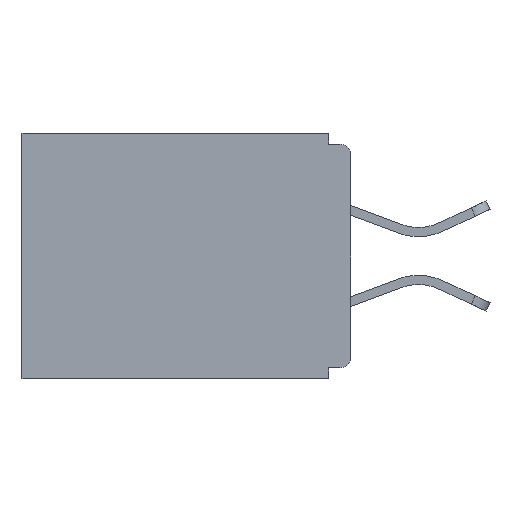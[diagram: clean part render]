
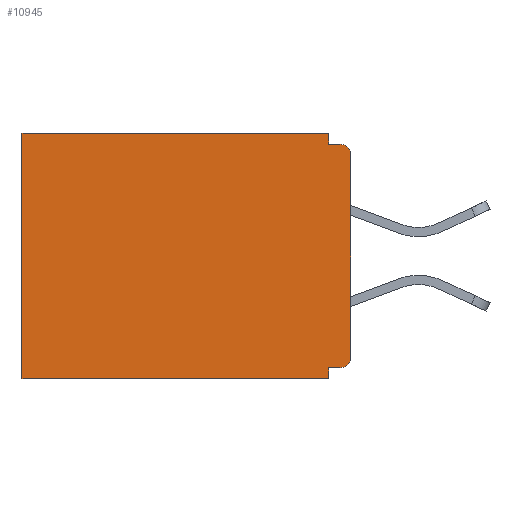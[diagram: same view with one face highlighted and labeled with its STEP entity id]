
A CAD part, left-side view. The second image highlights one B-rep face of the part: STEP entity #10945.
In plain terms, the highlighted planar face has unit normal (-1, 0, 0).
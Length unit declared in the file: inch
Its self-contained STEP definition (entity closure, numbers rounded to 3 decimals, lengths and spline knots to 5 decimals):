
#43 = AXIS2_PLACEMENT_3D ( 'NONE', #18187, #20463, #11558 ) ;
#1147 = CARTESIAN_POINT ( 'NONE',  ( 0.298, 0., -0.343 ) ) ;
#1182 = LINE ( 'NONE', #28851, #17991 ) ;
#1519 = EDGE_CURVE ( 'NONE', #20326, #28762, #3166, .T. ) ;
#1587 = LINE ( 'NONE', #18025, #18782 ) ;
#1724 = ORIENTED_EDGE ( 'NONE', *, *, #22339, .F. ) ;
#2515 = DIRECTION ( 'NONE',  ( 0., 0., -1. ) ) ;
#3166 = LINE ( 'NONE', #6079, #15088 ) ;
#3562 = LINE ( 'NONE', #15911, #8822 ) ;
#3618 = VECTOR ( 'NONE', #20977, 39.37008 ) ;
#3961 = ORIENTED_EDGE ( 'NONE', *, *, #25768, .F. ) ;
#4178 = CARTESIAN_POINT ( 'NONE',  ( 0.298, 0.46, 0. ) ) ;
#4232 = EDGE_CURVE ( 'NONE', #9191, #28944, #1587, .T. ) ;
#4562 = CARTESIAN_POINT ( 'NONE',  ( 0.298, 0.015, -0.328 ) ) ;
#4910 = CARTESIAN_POINT ( 'NONE',  ( 0.298, 0.46, -0.343 ) ) ;
#5823 = ORIENTED_EDGE ( 'NONE', *, *, #20097, .F. ) ;
#6053 = LINE ( 'NONE', #25702, #3618 ) ;
#6079 = CARTESIAN_POINT ( 'NONE',  ( 0.298, 0., 0. ) ) ;
#6229 = DIRECTION ( 'NONE',  ( -1., 0., 0. ) ) ;
#6431 = VERTEX_POINT ( 'NONE', #21099 ) ;
#6627 = DIRECTION ( 'NONE',  ( 0., 0., -1. ) ) ;
#6836 = EDGE_CURVE ( 'NONE', #28762, #16890, #15283, .T. ) ;
#7555 = EDGE_LOOP ( 'NONE', ( #28119, #8310, #25436, #8797, #10883, #5823, #1724, #18919, #17850, #3961 ) ) ;
#7641 = VECTOR ( 'NONE', #24606, 39.37008 ) ;
#7887 = VECTOR ( 'NONE', #7920, 39.37008 ) ;
#7920 = DIRECTION ( 'NONE',  ( 0., 1., 0. ) ) ;
#7973 = EDGE_CURVE ( 'NONE', #12589, #15435, #6053, .T. ) ;
#8310 = ORIENTED_EDGE ( 'NONE', *, *, #7973, .F. ) ;
#8620 = DIRECTION ( 'NONE',  ( 0., 0., -1. ) ) ;
#8695 = CARTESIAN_POINT ( 'NONE',  ( 0.298, 0.031, 0. ) ) ;
#8797 = ORIENTED_EDGE ( 'NONE', *, *, #1519, .T. ) ;
#8822 = VECTOR ( 'NONE', #2515, 39.37008 ) ;
#9191 = VERTEX_POINT ( 'NONE', #4562 ) ;
#10883 = ORIENTED_EDGE ( 'NONE', *, *, #6836, .T. ) ;
#10903 = CARTESIAN_POINT ( 'NONE',  ( 0.298, 0.015, -0.015 ) ) ;
#10945 = ADVANCED_FACE ( 'NONE', ( #22767 ), #12918, .F. ) ;
#10976 = CARTESIAN_POINT ( 'NONE',  ( 0.298, 0.015, -0.313 ) ) ;
#11558 = DIRECTION ( 'NONE',  ( 0., 0., -1. ) ) ;
#12589 = VERTEX_POINT ( 'NONE', #26981 ) ;
#12918 = PLANE ( 'NONE',  #43 ) ;
#13243 = CARTESIAN_POINT ( 'NONE',  ( 0.298, 0.46, 0. ) ) ;
#13919 = CARTESIAN_POINT ( 'NONE',  ( 0.298, 0.031, -0.343 ) ) ;
#15088 = VECTOR ( 'NONE', #17456, 39.37008 ) ;
#15237 = LINE ( 'NONE', #1147, #7887 ) ;
#15283 = LINE ( 'NONE', #4178, #26570 ) ;
#15396 = DIRECTION ( 'NONE',  ( 0., 0., -1. ) ) ;
#15435 = VERTEX_POINT ( 'NONE', #10903 ) ;
#15453 = CARTESIAN_POINT ( 'NONE',  ( 0.298, 0., -0.313 ) ) ;
#15621 = CARTESIAN_POINT ( 'NONE',  ( 0.298, 0., 0. ) ) ;
#15911 = CARTESIAN_POINT ( 'NONE',  ( 0.298, 0.031, -0.343 ) ) ;
#16277 = AXIS2_PLACEMENT_3D ( 'NONE', #17709, #19512, #8620 ) ;
#16398 = CIRCLE ( 'NONE', #19941, 0.015 ) ;
#16890 = VERTEX_POINT ( 'NONE', #4910 ) ;
#17456 = DIRECTION ( 'NONE',  ( 0., 1., 0. ) ) ;
#17709 = CARTESIAN_POINT ( 'NONE',  ( 0.298, 0.015, -0.03 ) ) ;
#17850 = ORIENTED_EDGE ( 'NONE', *, *, #18031, .T. ) ;
#17991 = VECTOR ( 'NONE', #15396, 39.37008 ) ;
#18025 = CARTESIAN_POINT ( 'NONE',  ( 0.298, 0., -0.328 ) ) ;
#18031 = EDGE_CURVE ( 'NONE', #9191, #24103, #16398, .T. ) ;
#18187 = CARTESIAN_POINT ( 'NONE',  ( 0.298, 0., 0. ) ) ;
#18782 = VECTOR ( 'NONE', #27762, 39.37008 ) ;
#18919 = ORIENTED_EDGE ( 'NONE', *, *, #4232, .F. ) ;
#19273 = VERTEX_POINT ( 'NONE', #13919 ) ;
#19512 = DIRECTION ( 'NONE',  ( -1., 0., 0. ) ) ;
#19941 = AXIS2_PLACEMENT_3D ( 'NONE', #10976, #6229, #28804 ) ;
#20097 = EDGE_CURVE ( 'NONE', #19273, #16890, #15237, .T. ) ;
#20326 = VERTEX_POINT ( 'NONE', #8695 ) ;
#20463 = DIRECTION ( 'NONE',  ( 1., 0., 0. ) ) ;
#20754 = EDGE_CURVE ( 'NONE', #20326, #12589, #1182, .T. ) ;
#20977 = DIRECTION ( 'NONE',  ( 0., -1., 0. ) ) ;
#21099 = CARTESIAN_POINT ( 'NONE',  ( 0.298, 0., -0.03 ) ) ;
#22339 = EDGE_CURVE ( 'NONE', #28944, #19273, #3562, .T. ) ;
#22767 = FACE_OUTER_BOUND ( 'NONE', #7555, .T. ) ;
#24103 = VERTEX_POINT ( 'NONE', #15453 ) ;
#24606 = DIRECTION ( 'NONE',  ( 0., 0., -1. ) ) ;
#25358 = CIRCLE ( 'NONE', #16277, 0.015 ) ;
#25436 = ORIENTED_EDGE ( 'NONE', *, *, #20754, .F. ) ;
#25610 = LINE ( 'NONE', #15621, #7641 ) ;
#25702 = CARTESIAN_POINT ( 'NONE',  ( 0.298, 0., -0.015 ) ) ;
#25768 = EDGE_CURVE ( 'NONE', #6431, #24103, #25610, .T. ) ;
#25853 = EDGE_CURVE ( 'NONE', #6431, #15435, #25358, .T. ) ;
#26570 = VECTOR ( 'NONE', #6627, 39.37008 ) ;
#26981 = CARTESIAN_POINT ( 'NONE',  ( 0.298, 0.031, -0.015 ) ) ;
#27281 = CARTESIAN_POINT ( 'NONE',  ( 0.298, 0.031, -0.328 ) ) ;
#27762 = DIRECTION ( 'NONE',  ( 0., 1., 0. ) ) ;
#28119 = ORIENTED_EDGE ( 'NONE', *, *, #25853, .T. ) ;
#28762 = VERTEX_POINT ( 'NONE', #13243 ) ;
#28804 = DIRECTION ( 'NONE',  ( 0., 0., -1. ) ) ;
#28851 = CARTESIAN_POINT ( 'NONE',  ( 0.298, 0.031, -0.343 ) ) ;
#28944 = VERTEX_POINT ( 'NONE', #27281 ) ;
